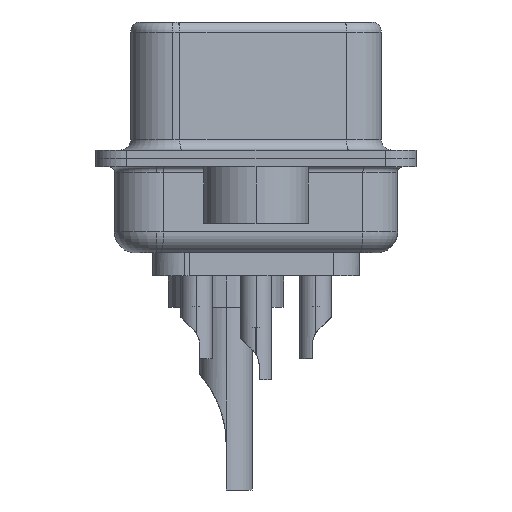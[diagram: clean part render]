
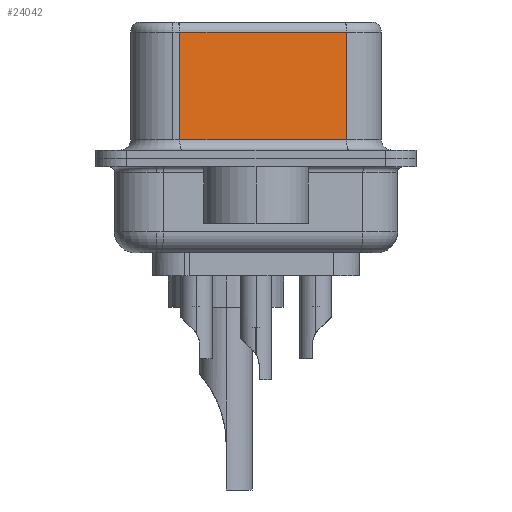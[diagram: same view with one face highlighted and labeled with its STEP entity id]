
A CAD part, left-side view. The second image highlights one B-rep face of the part: STEP entity #24042.
In plain terms, the highlighted planar face has unit normal (-0.985, -0.174, 0).
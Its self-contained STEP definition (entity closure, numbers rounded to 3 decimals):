
#646 = FACE_OUTER_BOUND ( 'NONE', #21562, .T. ) ;
#1276 = VECTOR ( 'NONE', #27617, 1000. ) ;
#4005 = ORIENTED_EDGE ( 'NONE', *, *, #22335, .T. ) ;
#4764 = CARTESIAN_POINT ( 'NONE',  ( 5.132, -4.322, 6.02 ) ) ;
#4922 = CARTESIAN_POINT ( 'NONE',  ( 3.73, 3.628, 6.52 ) ) ;
#5991 = ORIENTED_EDGE ( 'NONE', *, *, #26183, .T. ) ;
#6258 = CARTESIAN_POINT ( 'NONE',  ( 5.132, -4.322, 0.9 ) ) ;
#7368 = LINE ( 'NONE', #4764, #1276 ) ;
#8466 = VECTOR ( 'NONE', #21749, 1000. ) ;
#8739 = EDGE_CURVE ( 'NONE', #9696, #23777, #29833, .T. ) ;
#9696 = VERTEX_POINT ( 'NONE', #12257 ) ;
#10642 = ORIENTED_EDGE ( 'NONE', *, *, #21507, .T. ) ;
#11652 = PLANE ( 'NONE',  #20307 ) ;
#12148 = VECTOR ( 'NONE', #12806, 1000. ) ;
#12257 = CARTESIAN_POINT ( 'NONE',  ( 5.132, -4.322, 6.02 ) ) ;
#12806 = DIRECTION ( 'NONE',  ( 0., 0., -1. ) ) ;
#13396 = VERTEX_POINT ( 'NONE', #23972 ) ;
#14063 = DIRECTION ( 'NONE',  ( -0.174, 0.985, 0. ) ) ;
#14261 = CARTESIAN_POINT ( 'NONE',  ( 3.73, 3.628, 6.02 ) ) ;
#14474 = CARTESIAN_POINT ( 'NONE',  ( 5.132, -4.322, 0.9 ) ) ;
#15490 = LINE ( 'NONE', #4922, #24878 ) ;
#16590 = DIRECTION ( 'NONE',  ( 0., 0., -1. ) ) ;
#17039 = CARTESIAN_POINT ( 'NONE',  ( 5.132, -4.322, 6.52 ) ) ;
#20307 = AXIS2_PLACEMENT_3D ( 'NONE', #28075, #20730, #14063 ) ;
#20730 = DIRECTION ( 'NONE',  ( 0.985, 0.174, 0. ) ) ;
#20910 = ORIENTED_EDGE ( 'NONE', *, *, #8739, .F. ) ;
#21507 = EDGE_CURVE ( 'NONE', #13396, #23777, #22176, .T. ) ;
#21562 = EDGE_LOOP ( 'NONE', ( #20910, #5991, #4005, #10642 ) ) ;
#21749 = DIRECTION ( 'NONE',  ( 0.174, -0.985, 0. ) ) ;
#22176 = LINE ( 'NONE', #14474, #8466 ) ;
#22335 = EDGE_CURVE ( 'NONE', #22439, #13396, #15490, .T. ) ;
#22439 = VERTEX_POINT ( 'NONE', #14261 ) ;
#23777 = VERTEX_POINT ( 'NONE', #6258 ) ;
#23972 = CARTESIAN_POINT ( 'NONE',  ( 3.73, 3.628, 0.9 ) ) ;
#24042 = ADVANCED_FACE ( 'NONE', ( #646 ), #11652, .F. ) ;
#24878 = VECTOR ( 'NONE', #16590, 1000. ) ;
#26183 = EDGE_CURVE ( 'NONE', #9696, #22439, #7368, .T. ) ;
#27617 = DIRECTION ( 'NONE',  ( -0.174, 0.985, 0. ) ) ;
#28075 = CARTESIAN_POINT ( 'NONE',  ( 5.132, -4.322, 6.52 ) ) ;
#29833 = LINE ( 'NONE', #17039, #12148 ) ;
